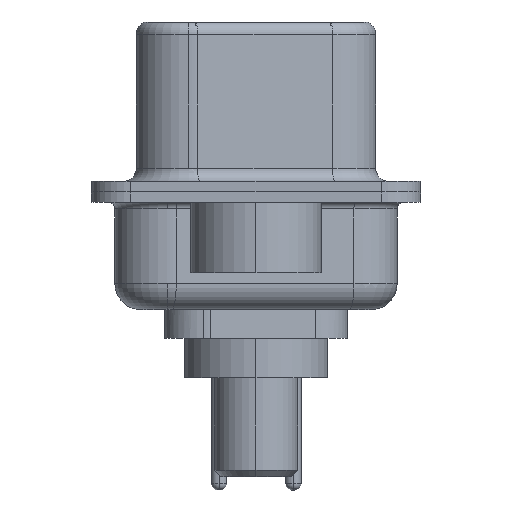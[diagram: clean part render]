
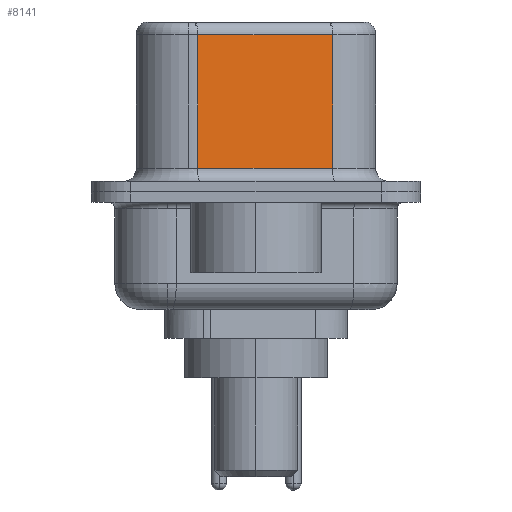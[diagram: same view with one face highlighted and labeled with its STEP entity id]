
A CAD part, left-side view. The second image highlights one B-rep face of the part: STEP entity #8141.
In plain terms, the highlighted planar face has unit normal (-0.985, -0.174, 0).
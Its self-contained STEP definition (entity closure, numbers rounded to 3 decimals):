
#1072 = EDGE_CURVE ( 'NONE', #17086, #3548, #14509, .T. ) ;
#2086 = DIRECTION ( 'NONE',  ( -0.174, 0.985, 0. ) ) ;
#2759 = CARTESIAN_POINT ( 'NONE',  ( 4.58, -2.927, 0.9 ) ) ;
#3106 = DIRECTION ( 'NONE',  ( -0.174, 0.985, 0. ) ) ;
#3243 = VECTOR ( 'NONE', #3106, 1000. ) ;
#3450 = CARTESIAN_POINT ( 'NONE',  ( 4.58, -2.927, 6.02 ) ) ;
#3548 = VERTEX_POINT ( 'NONE', #16330 ) ;
#4139 = ORIENTED_EDGE ( 'NONE', *, *, #11393, .T. ) ;
#4150 = VECTOR ( 'NONE', #12077, 1000. ) ;
#5304 = CARTESIAN_POINT ( 'NONE',  ( 4.58, -2.927, 6.02 ) ) ;
#6565 = PLANE ( 'NONE',  #9558 ) ;
#8141 = ADVANCED_FACE ( 'NONE', ( #19028 ), #6565, .F. ) ;
#8574 = LINE ( 'NONE', #10619, #4150 ) ;
#9558 = AXIS2_PLACEMENT_3D ( 'NONE', #16824, #10989, #2086 ) ;
#10038 = DIRECTION ( 'NONE',  ( 0.174, -0.985, 0. ) ) ;
#10293 = ORIENTED_EDGE ( 'NONE', *, *, #1072, .T. ) ;
#10619 = CARTESIAN_POINT ( 'NONE',  ( 4.58, -2.927, 6.52 ) ) ;
#10975 = CARTESIAN_POINT ( 'NONE',  ( 3.67, 2.233, 6.52 ) ) ;
#10989 = DIRECTION ( 'NONE',  ( 0.985, 0.174, 0. ) ) ;
#11393 = EDGE_CURVE ( 'NONE', #3548, #14918, #16560, .T. ) ;
#11416 = LINE ( 'NONE', #18842, #11867 ) ;
#11867 = VECTOR ( 'NONE', #10038, 1000. ) ;
#12077 = DIRECTION ( 'NONE',  ( 0., 0., -1. ) ) ;
#13463 = EDGE_CURVE ( 'NONE', #14918, #14804, #11416, .T. ) ;
#13868 = ORIENTED_EDGE ( 'NONE', *, *, #13463, .T. ) ;
#13958 = CARTESIAN_POINT ( 'NONE',  ( 3.67, 2.233, 0.9 ) ) ;
#14509 = LINE ( 'NONE', #5304, #3243 ) ;
#14804 = VERTEX_POINT ( 'NONE', #2759 ) ;
#14918 = VERTEX_POINT ( 'NONE', #13958 ) ;
#15127 = VECTOR ( 'NONE', #16875, 1000. ) ;
#16330 = CARTESIAN_POINT ( 'NONE',  ( 3.67, 2.233, 6.02 ) ) ;
#16467 = EDGE_CURVE ( 'NONE', #17086, #14804, #8574, .T. ) ;
#16560 = LINE ( 'NONE', #10975, #15127 ) ;
#16824 = CARTESIAN_POINT ( 'NONE',  ( 4.58, -2.927, 6.52 ) ) ;
#16875 = DIRECTION ( 'NONE',  ( 0., 0., -1. ) ) ;
#17086 = VERTEX_POINT ( 'NONE', #3450 ) ;
#17196 = ORIENTED_EDGE ( 'NONE', *, *, #16467, .F. ) ;
#18289 = EDGE_LOOP ( 'NONE', ( #17196, #10293, #4139, #13868 ) ) ;
#18842 = CARTESIAN_POINT ( 'NONE',  ( 4.58, -2.927, 0.9 ) ) ;
#19028 = FACE_OUTER_BOUND ( 'NONE', #18289, .T. ) ;
